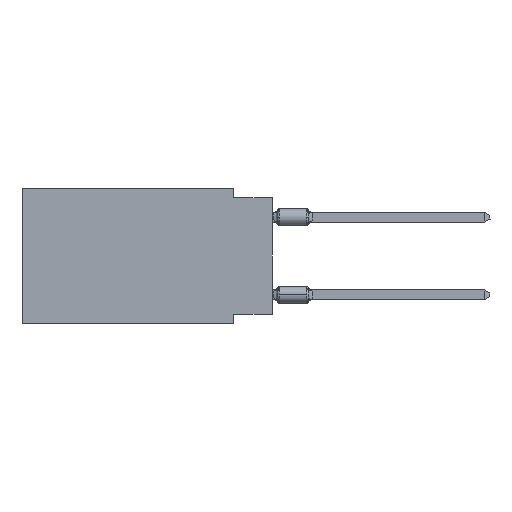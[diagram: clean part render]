
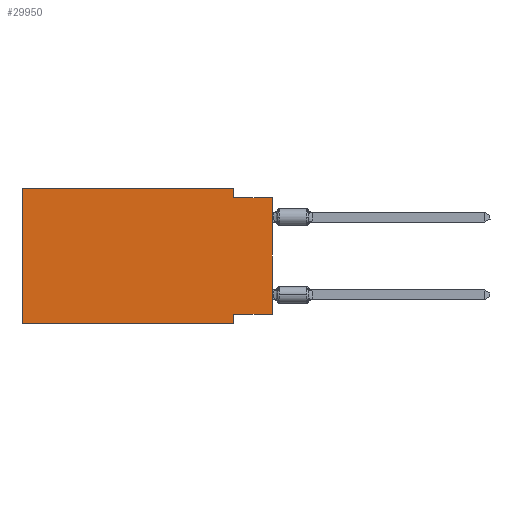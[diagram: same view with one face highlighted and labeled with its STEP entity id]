
A CAD part, left-side view. The second image highlights one B-rep face of the part: STEP entity #29950.
In plain terms, the highlighted planar face has unit normal (-1, 0, 0).
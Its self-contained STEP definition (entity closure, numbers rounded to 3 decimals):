
#687 = EDGE_CURVE ( 'NONE', #7732, #11528, #47554, .T. ) ;
#1597 = EDGE_LOOP ( 'NONE', ( #23356, #16007, #5839, #46370, #35284, #20497, #46989, #5969 ) ) ;
#1698 = CARTESIAN_POINT ( 'NONE',  ( 0., 0., -8.255 ) ) ;
#3161 = FACE_OUTER_BOUND ( 'NONE', #1597, .T. ) ;
#4403 = VERTEX_POINT ( 'NONE', #28392 ) ;
#5839 = ORIENTED_EDGE ( 'NONE', *, *, #10260, .F. ) ;
#5885 = CARTESIAN_POINT ( 'NONE',  ( 0., 0., -0.635 ) ) ;
#5969 = ORIENTED_EDGE ( 'NONE', *, *, #687, .F. ) ;
#6007 = LINE ( 'NONE', #38318, #46794 ) ;
#7093 = EDGE_CURVE ( 'NONE', #4403, #49915, #6007, .T. ) ;
#7593 = VECTOR ( 'NONE', #38433, 1000. ) ;
#7669 = LINE ( 'NONE', #20166, #49485 ) ;
#7732 = VERTEX_POINT ( 'NONE', #10227 ) ;
#10227 = CARTESIAN_POINT ( 'NONE',  ( 0., 0., -8.255 ) ) ;
#10260 = EDGE_CURVE ( 'NONE', #40559, #4403, #35533, .T. ) ;
#11528 = VERTEX_POINT ( 'NONE', #15025 ) ;
#13372 = DIRECTION ( 'NONE',  ( 0., -1., 0. ) ) ;
#14827 = CARTESIAN_POINT ( 'NONE',  ( 0., 16.383, 0. ) ) ;
#15025 = CARTESIAN_POINT ( 'NONE',  ( 0., 2.54, -8.255 ) ) ;
#16007 = ORIENTED_EDGE ( 'NONE', *, *, #7093, .F. ) ;
#16279 = EDGE_CURVE ( 'NONE', #7732, #49915, #17815, .T. ) ;
#16455 = EDGE_CURVE ( 'NONE', #48108, #46986, #23500, .T. ) ;
#17815 = LINE ( 'NONE', #46594, #7593 ) ;
#19493 = DIRECTION ( 'NONE',  ( 0., 0., -1. ) ) ;
#19593 = EDGE_CURVE ( 'NONE', #46986, #40559, #43692, .T. ) ;
#20166 = CARTESIAN_POINT ( 'NONE',  ( 0., 16.383, -8.89 ) ) ;
#20497 = ORIENTED_EDGE ( 'NONE', *, *, #53193, .T. ) ;
#21667 = DIRECTION ( 'NONE',  ( 0., 0., -1. ) ) ;
#23356 = ORIENTED_EDGE ( 'NONE', *, *, #16279, .T. ) ;
#23500 = LINE ( 'NONE', #14827, #44894 ) ;
#24031 = DIRECTION ( 'NONE',  ( 0., 0., 1. ) ) ;
#24364 = DIRECTION ( 'NONE',  ( 1., 0., 0. ) ) ;
#26274 = LINE ( 'NONE', #33354, #38488 ) ;
#27168 = CARTESIAN_POINT ( 'NONE',  ( 0., 2.54, 0. ) ) ;
#28392 = CARTESIAN_POINT ( 'NONE',  ( 0., 2.54, -0.635 ) ) ;
#29759 = EDGE_CURVE ( 'NONE', #11528, #42419, #26274, .T. ) ;
#29950 = ADVANCED_FACE ( 'NONE', ( #3161 ), #49600, .F. ) ;
#30715 = DIRECTION ( 'NONE',  ( 0., 1., 0. ) ) ;
#31587 = AXIS2_PLACEMENT_3D ( 'NONE', #45495, #24364, #36814 ) ;
#33354 = CARTESIAN_POINT ( 'NONE',  ( 0., 2.54, -8.89 ) ) ;
#34369 = CARTESIAN_POINT ( 'NONE',  ( 0., 16.383, 0. ) ) ;
#35029 = CARTESIAN_POINT ( 'NONE',  ( 0., 16.383, 0. ) ) ;
#35284 = ORIENTED_EDGE ( 'NONE', *, *, #16455, .F. ) ;
#35332 = CARTESIAN_POINT ( 'NONE',  ( 0., 2.54, -8.89 ) ) ;
#35533 = LINE ( 'NONE', #52120, #38377 ) ;
#35630 = DIRECTION ( 'NONE',  ( 0., -1., 0. ) ) ;
#36814 = DIRECTION ( 'NONE',  ( 0., 0., -1. ) ) ;
#38318 = CARTESIAN_POINT ( 'NONE',  ( 0., 0., -0.635 ) ) ;
#38377 = VECTOR ( 'NONE', #19493, 1000. ) ;
#38433 = DIRECTION ( 'NONE',  ( 0., 0., 1. ) ) ;
#38488 = VECTOR ( 'NONE', #21667, 1000. ) ;
#40559 = VERTEX_POINT ( 'NONE', #27168 ) ;
#40789 = VECTOR ( 'NONE', #30715, 1000. ) ;
#42419 = VERTEX_POINT ( 'NONE', #35332 ) ;
#43692 = LINE ( 'NONE', #35029, #47611 ) ;
#44894 = VECTOR ( 'NONE', #24031, 1000. ) ;
#45495 = CARTESIAN_POINT ( 'NONE',  ( 0., 16.383, 0. ) ) ;
#46370 = ORIENTED_EDGE ( 'NONE', *, *, #19593, .F. ) ;
#46594 = CARTESIAN_POINT ( 'NONE',  ( 0., 0., 0. ) ) ;
#46794 = VECTOR ( 'NONE', #13372, 1000. ) ;
#46986 = VERTEX_POINT ( 'NONE', #34369 ) ;
#46989 = ORIENTED_EDGE ( 'NONE', *, *, #29759, .F. ) ;
#47003 = DIRECTION ( 'NONE',  ( 0., -1., 0. ) ) ;
#47554 = LINE ( 'NONE', #1698, #40789 ) ;
#47611 = VECTOR ( 'NONE', #47003, 1000. ) ;
#48108 = VERTEX_POINT ( 'NONE', #49952 ) ;
#49485 = VECTOR ( 'NONE', #35630, 1000. ) ;
#49600 = PLANE ( 'NONE',  #31587 ) ;
#49915 = VERTEX_POINT ( 'NONE', #5885 ) ;
#49952 = CARTESIAN_POINT ( 'NONE',  ( 0., 16.383, -8.89 ) ) ;
#52120 = CARTESIAN_POINT ( 'NONE',  ( 0., 2.54, 0. ) ) ;
#53193 = EDGE_CURVE ( 'NONE', #48108, #42419, #7669, .T. ) ;
